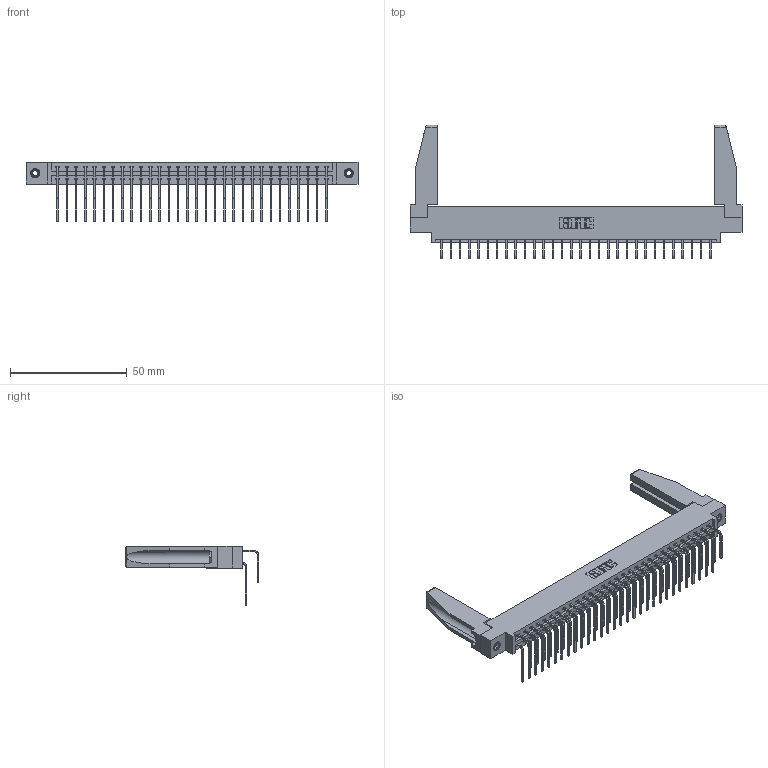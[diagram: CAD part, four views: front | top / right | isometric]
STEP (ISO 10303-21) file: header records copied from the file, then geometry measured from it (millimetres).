
FILE_DESCRIPTION (( 'STEP AP203' ), '1' );
FILE_NAME ('387-060-558-878.STEP', '2019-10-19T14:14:20', ( '' ), ( '' ), 'SwSTEP 2.0', 'SolidWorks 2016', '' );
FILE_SCHEMA (( 'CONFIG_CONTROL_DESIGN' ));
Length unit declared in the file: inch
Products named in the file (6): 345-292-001_558 559 Tail - 1; 387-060-558-878; 337 Part_0.170 Offset - 0.156 Dia-TI; 307-220-078; 345-250-001_345-250-001-102; 345-292-001_558 Tail - 2
Assembly tree (65 placements, depth 2):
  387-060-558-878
    337 Part_0.170 Offset - 0.156 Dia-TI
    345-292-001_558 559 Tail - 1  x30
    345-292-001_558 Tail - 2  x30
    345-250-001_345-250-001-102  x2
    307-220-078  x2
Bounding box: 141.88 x 56.96 x 25.53 mm (x, y, z)
Volume: 19015.1 mm3; surface area: 22541.9 mm2
Topology: 65 solids, 65 shells, 3608 faces, 10673 edges, 7026 vertices
Faces by surface type: plane 2558, cylinder 1034, cone 12, torus 4
Entity records: 29168 total; most frequent: CARTESIAN_POINT 4971, ORIENTED_EDGE 4812, DIRECTION 4238, EDGE_CURVE 2406, LINE 2200, VECTOR 2200, VERTEX_POINT 1596, AXIS2_PLACEMENT_3D 1019
